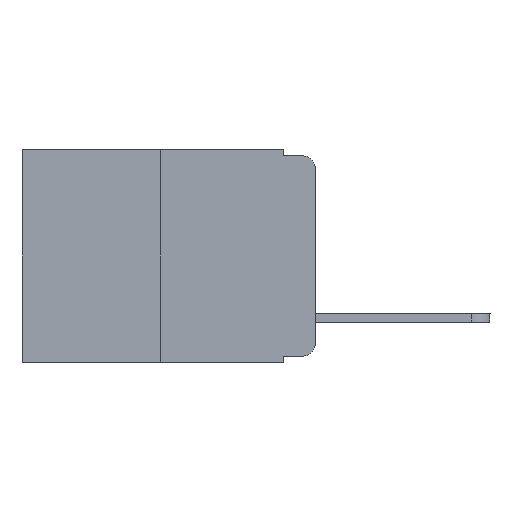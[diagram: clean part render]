
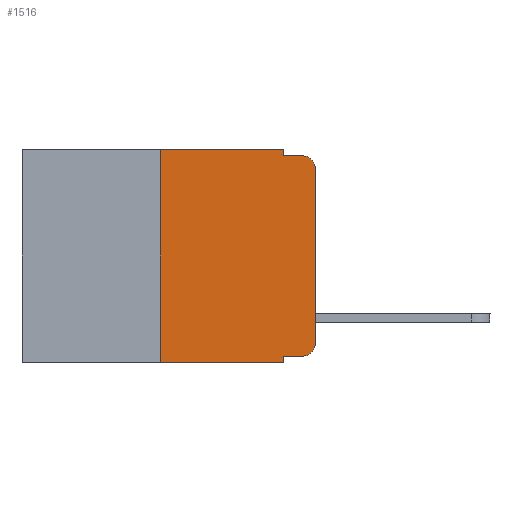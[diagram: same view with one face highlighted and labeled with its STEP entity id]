
A CAD part, left-side view. The second image highlights one B-rep face of the part: STEP entity #1516.
In plain terms, the highlighted planar face has unit normal (-1, 0, 0).
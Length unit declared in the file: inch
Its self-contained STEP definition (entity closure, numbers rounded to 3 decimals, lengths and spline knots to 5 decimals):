
#394 = VECTOR ( 'NONE', #18622, 39.37008 ) ;
#563 = VERTEX_POINT ( 'NONE', #12044 ) ;
#666 = AXIS2_PLACEMENT_3D ( 'NONE', #11383, #9187, #16662 ) ;
#838 = ORIENTED_EDGE ( 'NONE', *, *, #6496, .F. ) ;
#1059 = VERTEX_POINT ( 'NONE', #17520 ) ;
#1195 = LINE ( 'NONE', #14330, #12850 ) ;
#1516 = ADVANCED_FACE ( 'NONE', ( #21906 ), #23990, .F. ) ;
#1645 = CARTESIAN_POINT ( 'NONE',  ( 0., 0.02, -0.01 ) ) ;
#2197 = DIRECTION ( 'NONE',  ( 0., -1., 0. ) ) ;
#2219 = VECTOR ( 'NONE', #7430, 39.37008 ) ;
#2615 = LINE ( 'NONE', #22294, #23170 ) ;
#2749 = CARTESIAN_POINT ( 'NONE',  ( 0., 0.051, 0. ) ) ;
#3193 = DIRECTION ( 'NONE',  ( 1., 0., 0. ) ) ;
#3408 = VERTEX_POINT ( 'NONE', #17337 ) ;
#3845 = ORIENTED_EDGE ( 'NONE', *, *, #5276, .T. ) ;
#5276 = EDGE_CURVE ( 'NONE', #15318, #9159, #2615, .T. ) ;
#5686 = DIRECTION ( 'NONE',  ( -1., 0., 0. ) ) ;
#5812 = EDGE_CURVE ( 'NONE', #6032, #5931, #16062, .T. ) ;
#5931 = VERTEX_POINT ( 'NONE', #21686 ) ;
#6032 = VERTEX_POINT ( 'NONE', #20217 ) ;
#6444 = EDGE_CURVE ( 'NONE', #10203, #3408, #16645, .T. ) ;
#6496 = EDGE_CURVE ( 'NONE', #15318, #24040, #20546, .T. ) ;
#6898 = DIRECTION ( 'NONE',  ( 0., 0., -1. ) ) ;
#7344 = EDGE_CURVE ( 'NONE', #10203, #9159, #22414, .T. ) ;
#7430 = DIRECTION ( 'NONE',  ( 0., 0., 1. ) ) ;
#8397 = VECTOR ( 'NONE', #6898, 39.37008 ) ;
#8765 = EDGE_CURVE ( 'NONE', #5931, #14487, #21461, .T. ) ;
#8865 = ORIENTED_EDGE ( 'NONE', *, *, #5812, .T. ) ;
#8891 = AXIS2_PLACEMENT_3D ( 'NONE', #23503, #3193, #16033 ) ;
#9159 = VERTEX_POINT ( 'NONE', #10028 ) ;
#9187 = DIRECTION ( 'NONE',  ( -1., 0., 0. ) ) ;
#9316 = DIRECTION ( 'NONE',  ( 0., -1., 0. ) ) ;
#10028 = CARTESIAN_POINT ( 'NONE',  ( 0., 0.051, -0.343 ) ) ;
#10170 = ORIENTED_EDGE ( 'NONE', *, *, #8765, .T. ) ;
#10203 = VERTEX_POINT ( 'NONE', #18599 ) ;
#11254 = CARTESIAN_POINT ( 'NONE',  ( 0., 0.25, 0. ) ) ;
#11272 = LINE ( 'NONE', #22643, #17077 ) ;
#11383 = CARTESIAN_POINT ( 'NONE',  ( 0., 0.02, -0.313 ) ) ;
#12018 = CARTESIAN_POINT ( 'NONE',  ( 0., 0.25, 0. ) ) ;
#12044 = CARTESIAN_POINT ( 'NONE',  ( 0., 0.051, -0.01 ) ) ;
#12102 = ORIENTED_EDGE ( 'NONE', *, *, #6444, .T. ) ;
#12157 = DIRECTION ( 'NONE',  ( 0., 0., 1. ) ) ;
#12494 = DIRECTION ( 'NONE',  ( 0., -1., 0. ) ) ;
#12850 = VECTOR ( 'NONE', #12494, 39.37008 ) ;
#13928 = VECTOR ( 'NONE', #24111, 39.37008 ) ;
#14330 = CARTESIAN_POINT ( 'NONE',  ( 0., 0.051, -0.01 ) ) ;
#14487 = VERTEX_POINT ( 'NONE', #1645 ) ;
#14736 = VECTOR ( 'NONE', #12157, 39.37008 ) ;
#15116 = CIRCLE ( 'NONE', #666, 0.02 ) ;
#15318 = VERTEX_POINT ( 'NONE', #20092 ) ;
#15848 = LINE ( 'NONE', #2749, #8397 ) ;
#16023 = EDGE_CURVE ( 'NONE', #1059, #563, #15848, .T. ) ;
#16033 = DIRECTION ( 'NONE',  ( 0., 0., -1. ) ) ;
#16062 = LINE ( 'NONE', #23529, #14736 ) ;
#16392 = AXIS2_PLACEMENT_3D ( 'NONE', #22456, #5686, #20977 ) ;
#16645 = LINE ( 'NONE', #22021, #13928 ) ;
#16662 = DIRECTION ( 'NONE',  ( 0., 0., -1. ) ) ;
#17077 = VECTOR ( 'NONE', #2197, 39.37008 ) ;
#17337 = CARTESIAN_POINT ( 'NONE',  ( 0., 0.02, -0.333 ) ) ;
#17520 = CARTESIAN_POINT ( 'NONE',  ( 0., 0.051, 0. ) ) ;
#17584 = ORIENTED_EDGE ( 'NONE', *, *, #19215, .F. ) ;
#18599 = CARTESIAN_POINT ( 'NONE',  ( 0., 0.051, -0.333 ) ) ;
#18622 = DIRECTION ( 'NONE',  ( 0., 0., -1. ) ) ;
#19215 = EDGE_CURVE ( 'NONE', #24040, #1059, #11272, .T. ) ;
#19264 = EDGE_CURVE ( 'NONE', #3408, #6032, #15116, .T. ) ;
#19546 = ORIENTED_EDGE ( 'NONE', *, *, #20845, .F. ) ;
#19676 = EDGE_LOOP ( 'NONE', ( #8865, #10170, #19546, #21923, #17584, #838, #3845, #22733, #12102, #21159 ) ) ;
#20092 = CARTESIAN_POINT ( 'NONE',  ( 0., 0.25, -0.343 ) ) ;
#20217 = CARTESIAN_POINT ( 'NONE',  ( 0., 0., -0.313 ) ) ;
#20337 = CARTESIAN_POINT ( 'NONE',  ( 0., 0.051, 0. ) ) ;
#20546 = LINE ( 'NONE', #11254, #2219 ) ;
#20845 = EDGE_CURVE ( 'NONE', #563, #14487, #1195, .T. ) ;
#20977 = DIRECTION ( 'NONE',  ( 0., 0., -1. ) ) ;
#21159 = ORIENTED_EDGE ( 'NONE', *, *, #19264, .T. ) ;
#21461 = CIRCLE ( 'NONE', #16392, 0.02 ) ;
#21686 = CARTESIAN_POINT ( 'NONE',  ( 0., 0., -0.03 ) ) ;
#21906 = FACE_OUTER_BOUND ( 'NONE', #19676, .T. ) ;
#21923 = ORIENTED_EDGE ( 'NONE', *, *, #16023, .F. ) ;
#22021 = CARTESIAN_POINT ( 'NONE',  ( 0., 0.051, -0.333 ) ) ;
#22294 = CARTESIAN_POINT ( 'NONE',  ( 0., 0.473, -0.343 ) ) ;
#22414 = LINE ( 'NONE', #20337, #394 ) ;
#22456 = CARTESIAN_POINT ( 'NONE',  ( 0., 0.02, -0.03 ) ) ;
#22643 = CARTESIAN_POINT ( 'NONE',  ( 0., 0.473, 0. ) ) ;
#22733 = ORIENTED_EDGE ( 'NONE', *, *, #7344, .F. ) ;
#23170 = VECTOR ( 'NONE', #9316, 39.37008 ) ;
#23503 = CARTESIAN_POINT ( 'NONE',  ( 0., 0.473, 0. ) ) ;
#23529 = CARTESIAN_POINT ( 'NONE',  ( 0., 0., 0. ) ) ;
#23990 = PLANE ( 'NONE',  #8891 ) ;
#24040 = VERTEX_POINT ( 'NONE', #12018 ) ;
#24111 = DIRECTION ( 'NONE',  ( 0., -1., 0. ) ) ;
